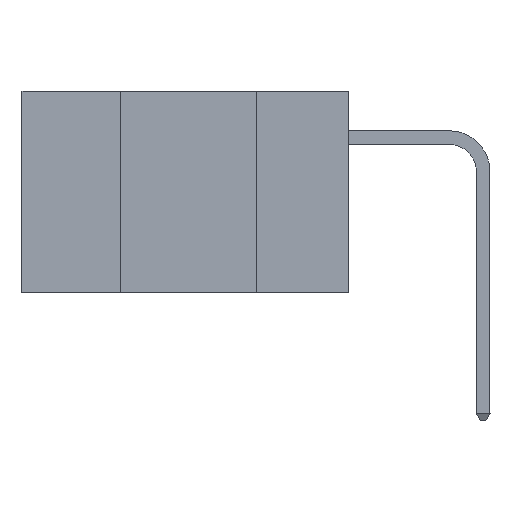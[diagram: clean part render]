
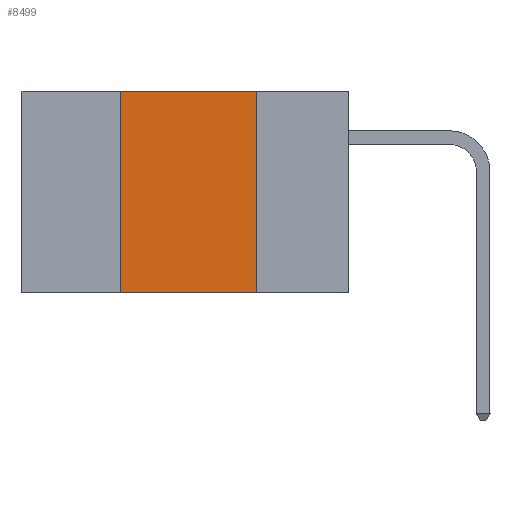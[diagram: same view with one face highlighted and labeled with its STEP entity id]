
A CAD part, left-side view. The second image highlights one B-rep face of the part: STEP entity #8499.
In plain terms, the highlighted planar face has unit normal (-1, 0, 0).
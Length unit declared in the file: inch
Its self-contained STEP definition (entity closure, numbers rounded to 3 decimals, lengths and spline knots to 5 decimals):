
#16 = AXIS2_PLACEMENT_3D ( 'NONE', #5000, #17135, #1973 ) ;
#1837 = LINE ( 'NONE', #4672, #8819 ) ;
#1973 = DIRECTION ( 'NONE',  ( 0., 0., -1. ) ) ;
#3027 = CARTESIAN_POINT ( 'NONE',  ( 0., 0.42, 0. ) ) ;
#3125 = CARTESIAN_POINT ( 'NONE',  ( 0., 0.42, 0. ) ) ;
#3440 = FACE_OUTER_BOUND ( 'NONE', #15272, .T. ) ;
#3527 = DIRECTION ( 'NONE',  ( 0., -1., 0. ) ) ;
#3781 = ORIENTED_EDGE ( 'NONE', *, *, #14080, .T. ) ;
#4382 = VERTEX_POINT ( 'NONE', #3027 ) ;
#4672 = CARTESIAN_POINT ( 'NONE',  ( 0., 0.17, 0. ) ) ;
#4692 = CARTESIAN_POINT ( 'NONE',  ( 0., 0.6, -0.37 ) ) ;
#5000 = CARTESIAN_POINT ( 'NONE',  ( 0., 0.6, 0. ) ) ;
#5092 = CARTESIAN_POINT ( 'NONE',  ( 0., 0.6, 0. ) ) ;
#5564 = CARTESIAN_POINT ( 'NONE',  ( 0., 0.42, -0.37 ) ) ;
#5729 = CARTESIAN_POINT ( 'NONE',  ( 0., 0.17, -0.37 ) ) ;
#5810 = VERTEX_POINT ( 'NONE', #9625 ) ;
#6356 = PLANE ( 'NONE',  #16 ) ;
#7511 = LINE ( 'NONE', #4692, #12920 ) ;
#8499 = ADVANCED_FACE ( 'NONE', ( #3440 ), #6356, .F. ) ;
#8589 = ORIENTED_EDGE ( 'NONE', *, *, #11199, .F. ) ;
#8819 = VECTOR ( 'NONE', #11700, 39.37008 ) ;
#9625 = CARTESIAN_POINT ( 'NONE',  ( 0., 0.17, 0. ) ) ;
#10338 = LINE ( 'NONE', #3125, #16722 ) ;
#11199 = EDGE_CURVE ( 'NONE', #4382, #5810, #16035, .T. ) ;
#11700 = DIRECTION ( 'NONE',  ( 0., 0., -1. ) ) ;
#12738 = DIRECTION ( 'NONE',  ( 0., -1., 0. ) ) ;
#12920 = VECTOR ( 'NONE', #12738, 39.37008 ) ;
#13166 = VERTEX_POINT ( 'NONE', #5564 ) ;
#13550 = VERTEX_POINT ( 'NONE', #5729 ) ;
#13815 = ORIENTED_EDGE ( 'NONE', *, *, #15759, .F. ) ;
#14080 = EDGE_CURVE ( 'NONE', #13166, #13550, #7511, .T. ) ;
#14439 = ORIENTED_EDGE ( 'NONE', *, *, #17058, .F. ) ;
#15272 = EDGE_LOOP ( 'NONE', ( #13815, #8589, #14439, #3781 ) ) ;
#15759 = EDGE_CURVE ( 'NONE', #5810, #13550, #1837, .T. ) ;
#15835 = VECTOR ( 'NONE', #3527, 39.37008 ) ;
#16035 = LINE ( 'NONE', #5092, #15835 ) ;
#16722 = VECTOR ( 'NONE', #17260, 39.37008 ) ;
#17058 = EDGE_CURVE ( 'NONE', #13166, #4382, #10338, .T. ) ;
#17135 = DIRECTION ( 'NONE',  ( 1., 0., 0. ) ) ;
#17260 = DIRECTION ( 'NONE',  ( 0., 0., 1. ) ) ;
